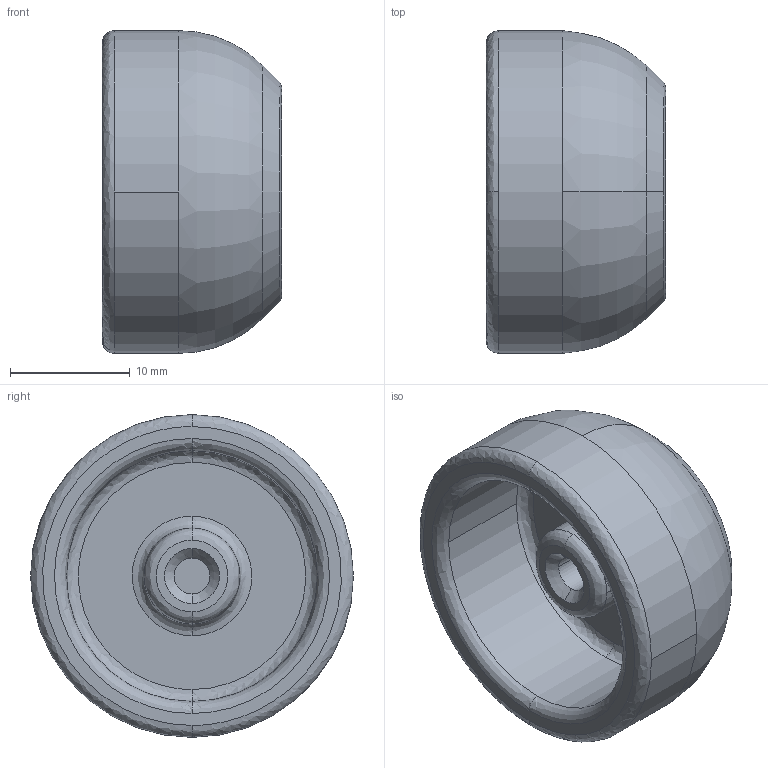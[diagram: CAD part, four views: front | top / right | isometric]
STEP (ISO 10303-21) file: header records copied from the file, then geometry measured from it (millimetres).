
FILE_DESCRIPTION (( 'STEP AP203' ), '1' );
FILE_NAME ('MOD9_V3__Hyd_Shock_Head.STEP', '2020-12-23T18:52:48', ( '' ), ( '' ), 'SwSTEP 2.0', 'SolidWorks 2019', '' );
FILE_SCHEMA (( 'CONFIG_CONTROL_DESIGN' ));
Length unit declared in the file: millimetre
Products named in the file (1): MOD9_V3__Hyd_Shock_Head
Bounding box: 15 x 27 x 27 mm (x, y, z)
Volume: 4397.6 mm3; surface area: 2880.1 mm2
Topology: 1 solids, 1 shells, 31 faces, 74 edges, 48 vertices
Faces by surface type: bspline 10, cylinder 8, cone 6, plane 5, torus 2
Entity records: 1589 total; most frequent: CARTESIAN_POINT 804, DIRECTION 158, ORIENTED_EDGE 148, EDGE_CURVE 74, AXIS2_PLACEMENT_3D 72, CIRCLE 50, VERTEX_POINT 48, EDGE_LOOP 34
